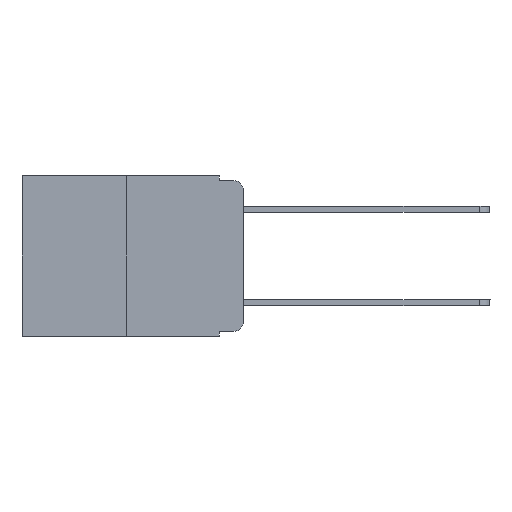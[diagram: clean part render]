
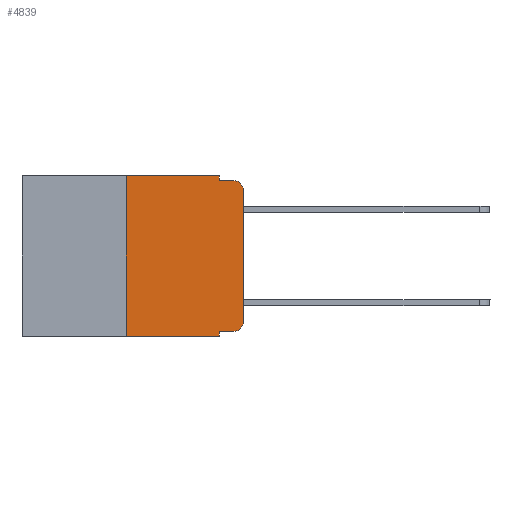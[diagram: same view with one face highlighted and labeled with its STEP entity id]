
A CAD part, left-side view. The second image highlights one B-rep face of the part: STEP entity #4839.
In plain terms, the highlighted planar face has unit normal (-1, 0, 0).
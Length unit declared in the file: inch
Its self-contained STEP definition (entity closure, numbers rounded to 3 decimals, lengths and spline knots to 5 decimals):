
#180 = FACE_OUTER_BOUND ( 'NONE', #4918, .T. ) ;
#457 = CARTESIAN_POINT ( 'NONE',  ( 0., 0.02, -0.01 ) ) ;
#853 = VERTEX_POINT ( 'NONE', #12649 ) ;
#1115 = VERTEX_POINT ( 'NONE', #2705 ) ;
#1294 = ORIENTED_EDGE ( 'NONE', *, *, #7515, .F. ) ;
#1424 = DIRECTION ( 'NONE',  ( 0., 0., -1. ) ) ;
#1679 = EDGE_CURVE ( 'NONE', #3829, #4322, #2830, .T. ) ;
#1691 = VERTEX_POINT ( 'NONE', #4609 ) ;
#1783 = CARTESIAN_POINT ( 'NONE',  ( 0., 0.051, -0.01 ) ) ;
#1899 = VECTOR ( 'NONE', #13534, 39.37008 ) ;
#2016 = CARTESIAN_POINT ( 'NONE',  ( 0., 0.25, -0.343 ) ) ;
#2040 = ORIENTED_EDGE ( 'NONE', *, *, #6550, .F. ) ;
#2101 = VECTOR ( 'NONE', #7907, 39.37008 ) ;
#2122 = AXIS2_PLACEMENT_3D ( 'NONE', #4401, #5442, #11742 ) ;
#2376 = VERTEX_POINT ( 'NONE', #2016 ) ;
#2406 = AXIS2_PLACEMENT_3D ( 'NONE', #11563, #12635, #8315 ) ;
#2485 = EDGE_CURVE ( 'NONE', #2878, #1115, #2975, .T. ) ;
#2705 = CARTESIAN_POINT ( 'NONE',  ( 0., 0.051, 0. ) ) ;
#2775 = VECTOR ( 'NONE', #1424, 39.37008 ) ;
#2830 = LINE ( 'NONE', #6733, #6237 ) ;
#2878 = VERTEX_POINT ( 'NONE', #13131 ) ;
#2975 = LINE ( 'NONE', #9523, #4306 ) ;
#3528 = ORIENTED_EDGE ( 'NONE', *, *, #8661, .F. ) ;
#3829 = VERTEX_POINT ( 'NONE', #4169 ) ;
#3846 = LINE ( 'NONE', #12086, #9721 ) ;
#4169 = CARTESIAN_POINT ( 'NONE',  ( 0., 0., -0.313 ) ) ;
#4306 = VECTOR ( 'NONE', #5384, 39.37008 ) ;
#4322 = VERTEX_POINT ( 'NONE', #6361 ) ;
#4401 = CARTESIAN_POINT ( 'NONE',  ( 0., 0.02, -0.03 ) ) ;
#4609 = CARTESIAN_POINT ( 'NONE',  ( 0., 0.051, -0.333 ) ) ;
#4662 = DIRECTION ( 'NONE',  ( 0., -1., 0. ) ) ;
#4709 = CARTESIAN_POINT ( 'NONE',  ( 0., 0.051, 0. ) ) ;
#4739 = VECTOR ( 'NONE', #4662, 39.37008 ) ;
#4839 = ADVANCED_FACE ( 'NONE', ( #180 ), #9323, .F. ) ;
#4918 = EDGE_LOOP ( 'NONE', ( #5483, #12818, #2040, #1294, #5519, #3528, #12147, #8654, #5137, #9463 ) ) ;
#4944 = CARTESIAN_POINT ( 'NONE',  ( 0., 0.25, 0. ) ) ;
#5137 = ORIENTED_EDGE ( 'NONE', *, *, #12845, .T. ) ;
#5146 = CARTESIAN_POINT ( 'NONE',  ( 0., 0.051, 0. ) ) ;
#5288 = VERTEX_POINT ( 'NONE', #457 ) ;
#5384 = DIRECTION ( 'NONE',  ( 0., -1., 0. ) ) ;
#5442 = DIRECTION ( 'NONE',  ( -1., 0., 0. ) ) ;
#5483 = ORIENTED_EDGE ( 'NONE', *, *, #1679, .T. ) ;
#5519 = ORIENTED_EDGE ( 'NONE', *, *, #2485, .F. ) ;
#5523 = LINE ( 'NONE', #11167, #2101 ) ;
#5541 = LINE ( 'NONE', #4709, #2775 ) ;
#5932 = AXIS2_PLACEMENT_3D ( 'NONE', #8686, #9742, #9891 ) ;
#6237 = VECTOR ( 'NONE', #7785, 39.37008 ) ;
#6295 = EDGE_CURVE ( 'NONE', #13323, #3829, #9735, .T. ) ;
#6361 = CARTESIAN_POINT ( 'NONE',  ( 0., 0., -0.03 ) ) ;
#6536 = LINE ( 'NONE', #4944, #13162 ) ;
#6550 = EDGE_CURVE ( 'NONE', #12225, #5288, #3846, .T. ) ;
#6733 = CARTESIAN_POINT ( 'NONE',  ( 0., 0., 0. ) ) ;
#7250 = LINE ( 'NONE', #5146, #1899 ) ;
#7515 = EDGE_CURVE ( 'NONE', #1115, #12225, #7250, .T. ) ;
#7785 = DIRECTION ( 'NONE',  ( 0., 0., 1. ) ) ;
#7874 = DIRECTION ( 'NONE',  ( 0., -1., 0. ) ) ;
#7907 = DIRECTION ( 'NONE',  ( 0., -1., 0. ) ) ;
#8066 = DIRECTION ( 'NONE',  ( 0., 0., 1. ) ) ;
#8315 = DIRECTION ( 'NONE',  ( 0., 0., -1. ) ) ;
#8485 = CARTESIAN_POINT ( 'NONE',  ( 0., 0.02, -0.333 ) ) ;
#8654 = ORIENTED_EDGE ( 'NONE', *, *, #9530, .F. ) ;
#8661 = EDGE_CURVE ( 'NONE', #2376, #2878, #6536, .T. ) ;
#8686 = CARTESIAN_POINT ( 'NONE',  ( 0., 0.02, -0.313 ) ) ;
#8884 = CARTESIAN_POINT ( 'NONE',  ( 0., 0.473, -0.343 ) ) ;
#9323 = PLANE ( 'NONE',  #2406 ) ;
#9463 = ORIENTED_EDGE ( 'NONE', *, *, #6295, .T. ) ;
#9523 = CARTESIAN_POINT ( 'NONE',  ( 0., 0.473, 0. ) ) ;
#9530 = EDGE_CURVE ( 'NONE', #1691, #853, #5541, .T. ) ;
#9572 = EDGE_CURVE ( 'NONE', #2376, #853, #9780, .T. ) ;
#9721 = VECTOR ( 'NONE', #7874, 39.37008 ) ;
#9735 = CIRCLE ( 'NONE', #5932, 0.02 ) ;
#9742 = DIRECTION ( 'NONE',  ( -1., 0., 0. ) ) ;
#9780 = LINE ( 'NONE', #8884, #4739 ) ;
#9891 = DIRECTION ( 'NONE',  ( 0., 0., -1. ) ) ;
#9936 = CIRCLE ( 'NONE', #2122, 0.02 ) ;
#11167 = CARTESIAN_POINT ( 'NONE',  ( 0., 0.051, -0.333 ) ) ;
#11563 = CARTESIAN_POINT ( 'NONE',  ( 0., 0.473, 0. ) ) ;
#11742 = DIRECTION ( 'NONE',  ( 0., 0., -1. ) ) ;
#12086 = CARTESIAN_POINT ( 'NONE',  ( 0., 0.051, -0.01 ) ) ;
#12147 = ORIENTED_EDGE ( 'NONE', *, *, #9572, .T. ) ;
#12225 = VERTEX_POINT ( 'NONE', #1783 ) ;
#12635 = DIRECTION ( 'NONE',  ( 1., 0., 0. ) ) ;
#12649 = CARTESIAN_POINT ( 'NONE',  ( 0., 0.051, -0.343 ) ) ;
#12818 = ORIENTED_EDGE ( 'NONE', *, *, #13280, .T. ) ;
#12845 = EDGE_CURVE ( 'NONE', #1691, #13323, #5523, .T. ) ;
#13131 = CARTESIAN_POINT ( 'NONE',  ( 0., 0.25, 0. ) ) ;
#13162 = VECTOR ( 'NONE', #8066, 39.37008 ) ;
#13280 = EDGE_CURVE ( 'NONE', #4322, #5288, #9936, .T. ) ;
#13323 = VERTEX_POINT ( 'NONE', #8485 ) ;
#13534 = DIRECTION ( 'NONE',  ( 0., 0., -1. ) ) ;
